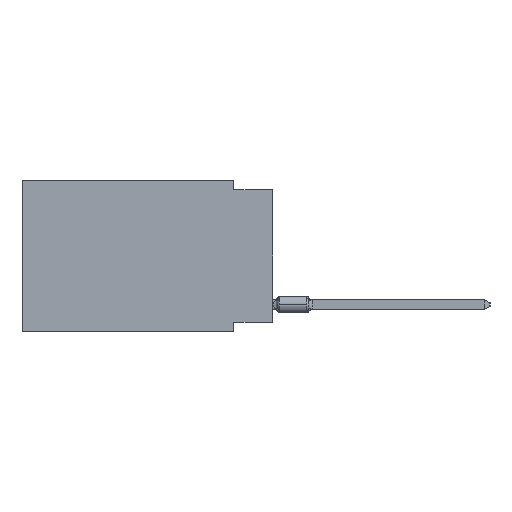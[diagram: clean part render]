
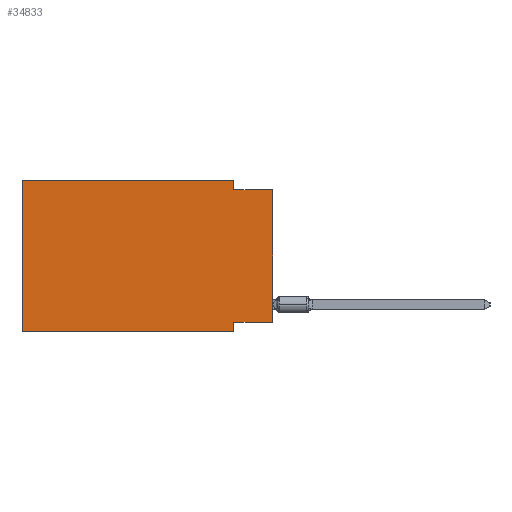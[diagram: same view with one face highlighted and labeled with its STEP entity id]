
A CAD part, left-side view. The second image highlights one B-rep face of the part: STEP entity #34833.
In plain terms, the highlighted planar face has unit normal (-1, 0, 0).
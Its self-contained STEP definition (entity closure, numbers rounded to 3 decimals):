
#25 = CARTESIAN_POINT ( 'NONE',  ( 0., 16.383, -9.906 ) ) ;
#107 = VERTEX_POINT ( 'NONE', #29527 ) ;
#2750 = EDGE_CURVE ( 'NONE', #34246, #107, #26806, .T. ) ;
#2905 = CARTESIAN_POINT ( 'NONE',  ( 0., 0., -9.271 ) ) ;
#3295 = CARTESIAN_POINT ( 'NONE',  ( 0., 0., 0. ) ) ;
#4082 = CARTESIAN_POINT ( 'NONE',  ( 0., 0., -9.271 ) ) ;
#5736 = DIRECTION ( 'NONE',  ( 0., 0., -1. ) ) ;
#6373 = CARTESIAN_POINT ( 'NONE',  ( 0., 0., -0.635 ) ) ;
#7091 = CARTESIAN_POINT ( 'NONE',  ( 0., 16.383, 0. ) ) ;
#7573 = CARTESIAN_POINT ( 'NONE',  ( 0., 2.54, 0. ) ) ;
#7656 = EDGE_CURVE ( 'NONE', #25958, #32571, #31427, .T. ) ;
#7817 = VECTOR ( 'NONE', #35629, 1000. ) ;
#8487 = DIRECTION ( 'NONE',  ( 1., 0., 0. ) ) ;
#10351 = CARTESIAN_POINT ( 'NONE',  ( 0., 0., -0.635 ) ) ;
#10728 = LINE ( 'NONE', #7573, #18869 ) ;
#11123 = EDGE_LOOP ( 'NONE', ( #34578, #13190, #11793, #17334, #29291, #30683, #31296, #29393 ) ) ;
#11793 = ORIENTED_EDGE ( 'NONE', *, *, #26766, .F. ) ;
#12340 = EDGE_CURVE ( 'NONE', #36366, #25958, #24270, .T. ) ;
#12391 = VECTOR ( 'NONE', #18019, 1000. ) ;
#12706 = CARTESIAN_POINT ( 'NONE',  ( 0., 16.383, -9.906 ) ) ;
#13190 = ORIENTED_EDGE ( 'NONE', *, *, #24183, .F. ) ;
#13691 = EDGE_CURVE ( 'NONE', #18879, #34246, #23546, .T. ) ;
#14541 = AXIS2_PLACEMENT_3D ( 'NONE', #33206, #8487, #5736 ) ;
#14592 = VECTOR ( 'NONE', #36834, 1000. ) ;
#16017 = CARTESIAN_POINT ( 'NONE',  ( 0., 16.383, 0. ) ) ;
#16495 = EDGE_CURVE ( 'NONE', #18879, #22617, #29420, .T. ) ;
#16735 = VECTOR ( 'NONE', #37117, 1000. ) ;
#17334 = ORIENTED_EDGE ( 'NONE', *, *, #7656, .F. ) ;
#17573 = CARTESIAN_POINT ( 'NONE',  ( 0., 2.54, -9.906 ) ) ;
#18019 = DIRECTION ( 'NONE',  ( 0., 0., 1. ) ) ;
#18243 = CARTESIAN_POINT ( 'NONE',  ( 0., 2.54, -9.271 ) ) ;
#18404 = LINE ( 'NONE', #12706, #14592 ) ;
#18869 = VECTOR ( 'NONE', #37022, 1000. ) ;
#18879 = VERTEX_POINT ( 'NONE', #4082 ) ;
#20590 = DIRECTION ( 'NONE',  ( 0., 1., 0. ) ) ;
#22617 = VERTEX_POINT ( 'NONE', #10351 ) ;
#23546 = LINE ( 'NONE', #2905, #32510 ) ;
#23611 = FACE_OUTER_BOUND ( 'NONE', #11123, .T. ) ;
#23889 = DIRECTION ( 'NONE',  ( 0., 0., 1. ) ) ;
#24183 = EDGE_CURVE ( 'NONE', #37778, #22617, #24248, .T. ) ;
#24248 = LINE ( 'NONE', #6373, #30110 ) ;
#24270 = LINE ( 'NONE', #24663, #33042 ) ;
#24663 = CARTESIAN_POINT ( 'NONE',  ( 0., 16.383, 0. ) ) ;
#25958 = VERTEX_POINT ( 'NONE', #16017 ) ;
#26766 = EDGE_CURVE ( 'NONE', #32571, #37778, #10728, .T. ) ;
#26806 = LINE ( 'NONE', #17573, #7817 ) ;
#27143 = PLANE ( 'NONE',  #14541 ) ;
#29291 = ORIENTED_EDGE ( 'NONE', *, *, #12340, .F. ) ;
#29393 = ORIENTED_EDGE ( 'NONE', *, *, #13691, .F. ) ;
#29420 = LINE ( 'NONE', #3295, #12391 ) ;
#29527 = CARTESIAN_POINT ( 'NONE',  ( 0., 2.54, -9.906 ) ) ;
#30110 = VECTOR ( 'NONE', #36013, 1000. ) ;
#30683 = ORIENTED_EDGE ( 'NONE', *, *, #35618, .T. ) ;
#31296 = ORIENTED_EDGE ( 'NONE', *, *, #2750, .F. ) ;
#31427 = LINE ( 'NONE', #7091, #16735 ) ;
#31859 = CARTESIAN_POINT ( 'NONE',  ( 0., 2.54, -0.635 ) ) ;
#32510 = VECTOR ( 'NONE', #20590, 1000. ) ;
#32571 = VERTEX_POINT ( 'NONE', #37067 ) ;
#33042 = VECTOR ( 'NONE', #23889, 1000. ) ;
#33206 = CARTESIAN_POINT ( 'NONE',  ( 0., 16.383, 0. ) ) ;
#34246 = VERTEX_POINT ( 'NONE', #18243 ) ;
#34578 = ORIENTED_EDGE ( 'NONE', *, *, #16495, .T. ) ;
#34833 = ADVANCED_FACE ( 'NONE', ( #23611 ), #27143, .F. ) ;
#35618 = EDGE_CURVE ( 'NONE', #36366, #107, #18404, .T. ) ;
#35629 = DIRECTION ( 'NONE',  ( 0., 0., -1. ) ) ;
#36013 = DIRECTION ( 'NONE',  ( 0., -1., 0. ) ) ;
#36366 = VERTEX_POINT ( 'NONE', #25 ) ;
#36834 = DIRECTION ( 'NONE',  ( 0., -1., 0. ) ) ;
#37022 = DIRECTION ( 'NONE',  ( 0., 0., -1. ) ) ;
#37067 = CARTESIAN_POINT ( 'NONE',  ( 0., 2.54, 0. ) ) ;
#37117 = DIRECTION ( 'NONE',  ( 0., -1., 0. ) ) ;
#37778 = VERTEX_POINT ( 'NONE', #31859 ) ;
